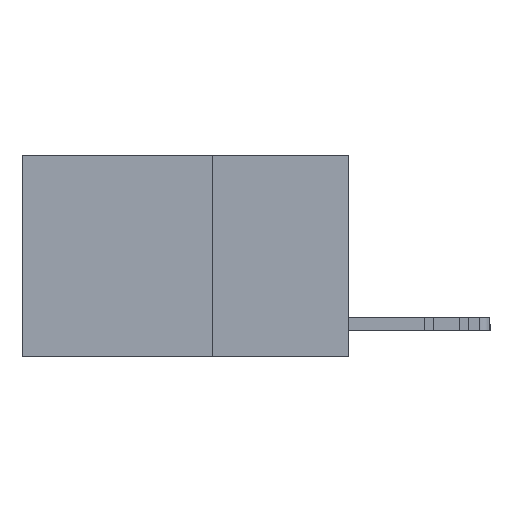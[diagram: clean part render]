
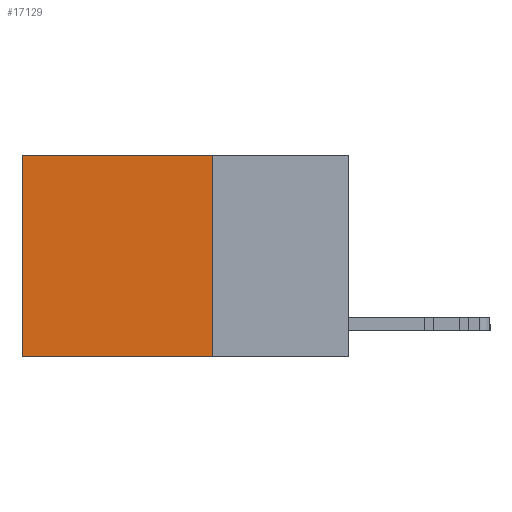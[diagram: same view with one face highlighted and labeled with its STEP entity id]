
A CAD part, left-side view. The second image highlights one B-rep face of the part: STEP entity #17129.
In plain terms, the highlighted planar face has unit normal (-1, 0, 0).
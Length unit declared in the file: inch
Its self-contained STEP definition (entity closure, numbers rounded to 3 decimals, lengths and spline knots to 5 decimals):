
#693 = ORIENTED_EDGE ( 'NONE', *, *, #26582, .T. ) ;
#726 = DIRECTION ( 'NONE',  ( 0., 0., -1. ) ) ;
#927 = VECTOR ( 'NONE', #21091, 39.37008 ) ;
#1015 = LINE ( 'NONE', #21904, #26979 ) ;
#1756 = CARTESIAN_POINT ( 'NONE',  ( 0.2625, 0.6, -0.37 ) ) ;
#2423 = VECTOR ( 'NONE', #12540, 39.37008 ) ;
#3918 = CARTESIAN_POINT ( 'NONE',  ( 0.2625, 0.25, -0.37 ) ) ;
#4122 = CARTESIAN_POINT ( 'NONE',  ( 0.2625, 0.25, 0. ) ) ;
#6068 = LINE ( 'NONE', #4122, #2423 ) ;
#7176 = EDGE_CURVE ( 'NONE', #11586, #12834, #1015, .T. ) ;
#9398 = LINE ( 'NONE', #18081, #9975 ) ;
#9975 = VECTOR ( 'NONE', #22110, 39.37008 ) ;
#10225 = LINE ( 'NONE', #10370, #927 ) ;
#10370 = CARTESIAN_POINT ( 'NONE',  ( 0.2625, 0.25, 0. ) ) ;
#10876 = ORIENTED_EDGE ( 'NONE', *, *, #20338, .F. ) ;
#11586 = VERTEX_POINT ( 'NONE', #24343 ) ;
#12540 = DIRECTION ( 'NONE',  ( 0., 1., 0. ) ) ;
#12834 = VERTEX_POINT ( 'NONE', #1756 ) ;
#13082 = VERTEX_POINT ( 'NONE', #24315 ) ;
#13408 = FACE_OUTER_BOUND ( 'NONE', #18309, .T. ) ;
#16013 = ORIENTED_EDGE ( 'NONE', *, *, #7176, .T. ) ;
#17129 = ADVANCED_FACE ( 'NONE', ( #13408 ), #23844, .F. ) ;
#17736 = DIRECTION ( 'NONE',  ( 1., 0., 0. ) ) ;
#18015 = VERTEX_POINT ( 'NONE', #3918 ) ;
#18081 = CARTESIAN_POINT ( 'NONE',  ( 0.2625, 0.25, -0.37 ) ) ;
#18309 = EDGE_LOOP ( 'NONE', ( #16013, #21784, #10876, #693 ) ) ;
#20338 = EDGE_CURVE ( 'NONE', #13082, #18015, #10225, .T. ) ;
#21091 = DIRECTION ( 'NONE',  ( 0., 0., -1. ) ) ;
#21784 = ORIENTED_EDGE ( 'NONE', *, *, #24328, .F. ) ;
#21904 = CARTESIAN_POINT ( 'NONE',  ( 0.2625, 0.6, 0. ) ) ;
#22110 = DIRECTION ( 'NONE',  ( 0., 1., 0. ) ) ;
#23530 = AXIS2_PLACEMENT_3D ( 'NONE', #25636, #17736, #726 ) ;
#23844 = PLANE ( 'NONE',  #23530 ) ;
#24315 = CARTESIAN_POINT ( 'NONE',  ( 0.2625, 0.25, 0. ) ) ;
#24328 = EDGE_CURVE ( 'NONE', #18015, #12834, #9398, .T. ) ;
#24343 = CARTESIAN_POINT ( 'NONE',  ( 0.2625, 0.6, 0. ) ) ;
#25636 = CARTESIAN_POINT ( 'NONE',  ( 0.2625, 0.25, 0. ) ) ;
#26472 = DIRECTION ( 'NONE',  ( 0., 0., -1. ) ) ;
#26582 = EDGE_CURVE ( 'NONE', #13082, #11586, #6068, .T. ) ;
#26979 = VECTOR ( 'NONE', #26472, 39.37008 ) ;
